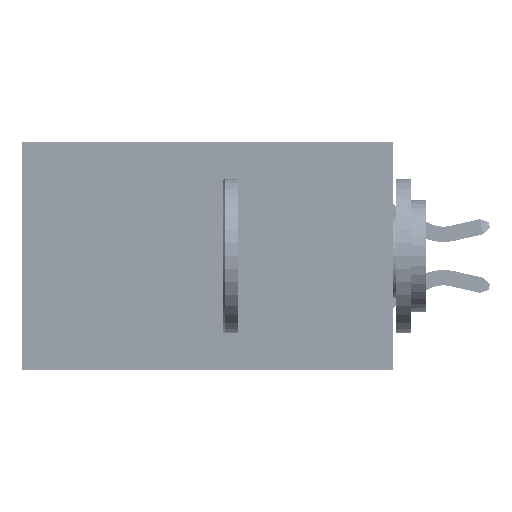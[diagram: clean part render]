
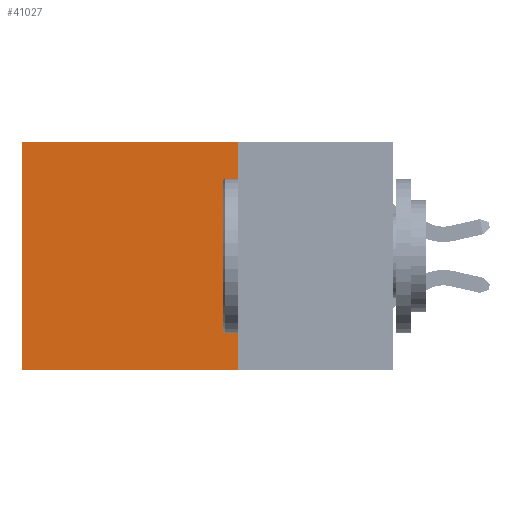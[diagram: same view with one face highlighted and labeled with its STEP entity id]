
A CAD part, left-side view. The second image highlights one B-rep face of the part: STEP entity #41027.
In plain terms, the highlighted planar face has unit normal (-1, 0, 0).
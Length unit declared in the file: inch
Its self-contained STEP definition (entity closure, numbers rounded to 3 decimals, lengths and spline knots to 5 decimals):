
#1189 = ORIENTED_EDGE ( 'NONE', *, *, #22983, .T. ) ;
#1815 = DIRECTION ( 'NONE',  ( 0., 1., 0. ) ) ;
#1993 = FACE_OUTER_BOUND ( 'NONE', #20559, .T. ) ;
#2777 = CARTESIAN_POINT ( 'NONE',  ( 0.2875, 0.25, -0.37 ) ) ;
#5231 = CARTESIAN_POINT ( 'NONE',  ( 0.2875, 0.25, 0. ) ) ;
#6329 = LINE ( 'NONE', #43326, #41544 ) ;
#8743 = CARTESIAN_POINT ( 'NONE',  ( 0.2875, 0.6, 0. ) ) ;
#9738 = VECTOR ( 'NONE', #11320, 39.37008 ) ;
#11320 = DIRECTION ( 'NONE',  ( 0., 1., 0. ) ) ;
#12429 = CARTESIAN_POINT ( 'NONE',  ( 0.2875, 0.6, -0.37 ) ) ;
#12900 = CARTESIAN_POINT ( 'NONE',  ( 0.2875, 0.6, 0. ) ) ;
#14448 = VERTEX_POINT ( 'NONE', #2777 ) ;
#15645 = CARTESIAN_POINT ( 'NONE',  ( 0.2875, 0.25, 0. ) ) ;
#18109 = VERTEX_POINT ( 'NONE', #12900 ) ;
#18577 = EDGE_CURVE ( 'NONE', #18109, #35246, #28519, .T. ) ;
#19506 = LINE ( 'NONE', #21608, #9738 ) ;
#20559 = EDGE_LOOP ( 'NONE', ( #22279, #29167, #20987, #1189 ) ) ;
#20987 = ORIENTED_EDGE ( 'NONE', *, *, #44296, .F. ) ;
#21608 = CARTESIAN_POINT ( 'NONE',  ( 0.2875, 0.25, 0. ) ) ;
#22279 = ORIENTED_EDGE ( 'NONE', *, *, #18577, .T. ) ;
#22983 = EDGE_CURVE ( 'NONE', #37958, #18109, #19506, .T. ) ;
#23029 = DIRECTION ( 'NONE',  ( 1., 0., 0. ) ) ;
#25560 = AXIS2_PLACEMENT_3D ( 'NONE', #15645, #23029, #36485 ) ;
#26576 = VECTOR ( 'NONE', #39779, 39.37008 ) ;
#28519 = LINE ( 'NONE', #8743, #34437 ) ;
#29167 = ORIENTED_EDGE ( 'NONE', *, *, #41094, .F. ) ;
#32938 = DIRECTION ( 'NONE',  ( 0., 0., -1. ) ) ;
#34437 = VECTOR ( 'NONE', #32938, 39.37008 ) ;
#35246 = VERTEX_POINT ( 'NONE', #12429 ) ;
#35737 = LINE ( 'NONE', #5231, #26576 ) ;
#36485 = DIRECTION ( 'NONE',  ( 0., 0., -1. ) ) ;
#37958 = VERTEX_POINT ( 'NONE', #44049 ) ;
#39779 = DIRECTION ( 'NONE',  ( 0., 0., -1. ) ) ;
#41027 = ADVANCED_FACE ( 'NONE', ( #1993 ), #43786, .F. ) ;
#41094 = EDGE_CURVE ( 'NONE', #14448, #35246, #6329, .T. ) ;
#41544 = VECTOR ( 'NONE', #1815, 39.37008 ) ;
#43326 = CARTESIAN_POINT ( 'NONE',  ( 0.2875, 0.25, -0.37 ) ) ;
#43786 = PLANE ( 'NONE',  #25560 ) ;
#44049 = CARTESIAN_POINT ( 'NONE',  ( 0.2875, 0.25, 0. ) ) ;
#44296 = EDGE_CURVE ( 'NONE', #37958, #14448, #35737, .T. ) ;
